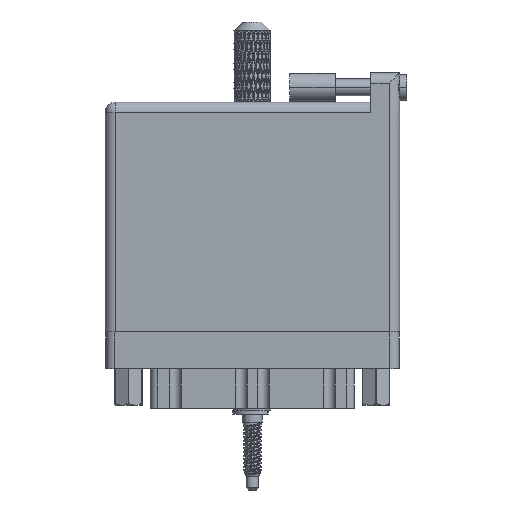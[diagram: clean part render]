
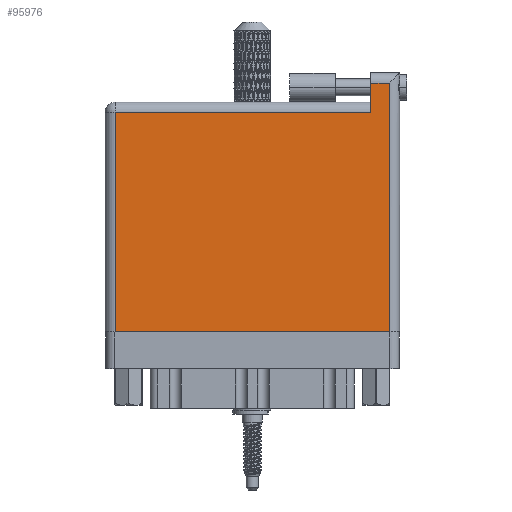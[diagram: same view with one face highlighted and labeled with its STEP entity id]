
A CAD part, front view. The second image highlights one B-rep face of the part: STEP entity #95976.
In plain terms, the highlighted face is planar.
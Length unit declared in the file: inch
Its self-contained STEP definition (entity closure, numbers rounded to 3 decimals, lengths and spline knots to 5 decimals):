
#737 = VERTEX_POINT ( 'NONE', #77389 ) ;
#2198 = DIRECTION ( 'NONE',  ( 0., -1., 0. ) ) ;
#7829 = VECTOR ( 'NONE', #98135, 39.37008 ) ;
#9385 = CARTESIAN_POINT ( 'NONE',  ( 0.07, 0., 0. ) ) ;
#10730 = EDGE_LOOP ( 'NONE', ( #78697, #86429, #100278, #36557, #108673, #95007 ) ) ;
#19349 = VECTOR ( 'NONE', #94966, 39.37008 ) ;
#19357 = VERTEX_POINT ( 'NONE', #21299 ) ;
#21299 = CARTESIAN_POINT ( 'NONE',  ( 1.938, 0., 0. ) ) ;
#22245 = EDGE_CURVE ( 'NONE', #737, #63990, #94436, .T. ) ;
#25634 = EDGE_CURVE ( 'NONE', #29740, #737, #48470, .T. ) ;
#26628 = VECTOR ( 'NONE', #40858, 39.37008 ) ;
#29740 = VERTEX_POINT ( 'NONE', #88711 ) ;
#31543 = VERTEX_POINT ( 'NONE', #76258 ) ;
#36557 = ORIENTED_EDGE ( 'NONE', *, *, #25634, .T. ) ;
#37490 = AXIS2_PLACEMENT_3D ( 'NONE', #97979, #66004, #64878 ) ;
#38870 = PLANE ( 'NONE',  #37490 ) ;
#40858 = DIRECTION ( 'NONE',  ( 0., 1., 0. ) ) ;
#41696 = VERTEX_POINT ( 'NONE', #49810 ) ;
#42853 = EDGE_CURVE ( 'NONE', #41696, #19357, #68461, .T. ) ;
#43398 = EDGE_CURVE ( 'NONE', #31543, #29740, #56093, .T. ) ;
#45275 = CARTESIAN_POINT ( 'NONE',  ( 0., 1.496, 0. ) ) ;
#48470 = LINE ( 'NONE', #108100, #7829 ) ;
#49810 = CARTESIAN_POINT ( 'NONE',  ( 0.07, 0., 0. ) ) ;
#51307 = DIRECTION ( 'NONE',  ( 1., 0., 0. ) ) ;
#54649 = EDGE_CURVE ( 'NONE', #63990, #41696, #61296, .T. ) ;
#56093 = LINE ( 'NONE', #107414, #107595 ) ;
#57166 = FACE_OUTER_BOUND ( 'NONE', #10730, .T. ) ;
#61296 = LINE ( 'NONE', #9385, #104369 ) ;
#63990 = VERTEX_POINT ( 'NONE', #84756 ) ;
#64878 = DIRECTION ( 'NONE',  ( -1., 0., 0. ) ) ;
#66004 = DIRECTION ( 'NONE',  ( 0., 0., -1. ) ) ;
#68461 = LINE ( 'NONE', #93243, #100465 ) ;
#76258 = CARTESIAN_POINT ( 'NONE',  ( 1.938, 1.696, 0. ) ) ;
#77389 = CARTESIAN_POINT ( 'NONE',  ( 1.811, 1.496, 0. ) ) ;
#78697 = ORIENTED_EDGE ( 'NONE', *, *, #42853, .T. ) ;
#84486 = LINE ( 'NONE', #107703, #26628 ) ;
#84756 = CARTESIAN_POINT ( 'NONE',  ( 0.07, 1.496, 0. ) ) ;
#86429 = ORIENTED_EDGE ( 'NONE', *, *, #91748, .T. ) ;
#88711 = CARTESIAN_POINT ( 'NONE',  ( 1.811, 1.696, 0. ) ) ;
#89203 = DIRECTION ( 'NONE',  ( -1., 0., 0. ) ) ;
#91748 = EDGE_CURVE ( 'NONE', #19357, #31543, #84486, .T. ) ;
#93243 = CARTESIAN_POINT ( 'NONE',  ( 0., 0., 0. ) ) ;
#94436 = LINE ( 'NONE', #45275, #19349 ) ;
#94966 = DIRECTION ( 'NONE',  ( -1., 0., 0. ) ) ;
#95007 = ORIENTED_EDGE ( 'NONE', *, *, #54649, .T. ) ;
#95976 = ADVANCED_FACE ( 'NONE', ( #57166 ), #38870, .F. ) ;
#97979 = CARTESIAN_POINT ( 'NONE',  ( 0., 1.566, 0. ) ) ;
#98135 = DIRECTION ( 'NONE',  ( 0., -1., 0. ) ) ;
#100278 = ORIENTED_EDGE ( 'NONE', *, *, #43398, .T. ) ;
#100465 = VECTOR ( 'NONE', #51307, 39.37008 ) ;
#104369 = VECTOR ( 'NONE', #2198, 39.37008 ) ;
#107414 = CARTESIAN_POINT ( 'NONE',  ( 0., 1.696, 0. ) ) ;
#107595 = VECTOR ( 'NONE', #89203, 39.37008 ) ;
#107703 = CARTESIAN_POINT ( 'NONE',  ( 1.938, 1.766, 0. ) ) ;
#108100 = CARTESIAN_POINT ( 'NONE',  ( 1.811, 1.766, 0. ) ) ;
#108673 = ORIENTED_EDGE ( 'NONE', *, *, #22245, .T. ) ;
